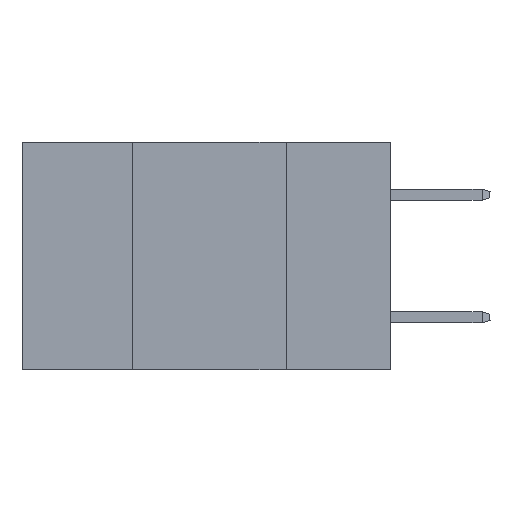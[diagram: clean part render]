
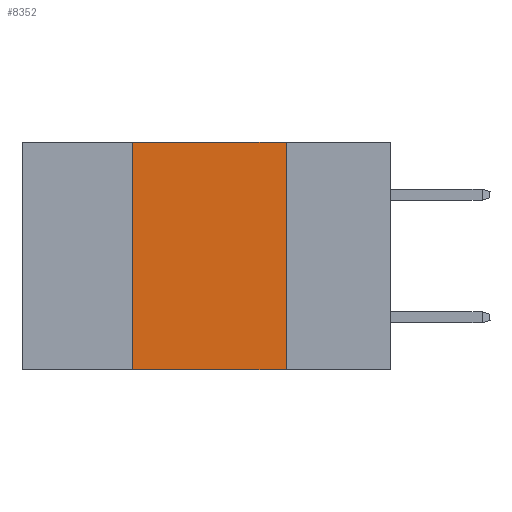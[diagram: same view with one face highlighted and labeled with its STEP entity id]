
A CAD part, left-side view. The second image highlights one B-rep face of the part: STEP entity #8352.
In plain terms, the highlighted planar face has unit normal (-1, 0, 0).
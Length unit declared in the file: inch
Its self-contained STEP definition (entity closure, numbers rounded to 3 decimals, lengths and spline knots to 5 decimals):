
#194 = ORIENTED_EDGE ( 'NONE', *, *, #8612, .T. ) ;
#572 = CARTESIAN_POINT ( 'NONE',  ( 0., 0.6, 0. ) ) ;
#630 = VECTOR ( 'NONE', #4818, 39.37008 ) ;
#926 = LINE ( 'NONE', #2051, #630 ) ;
#952 = VECTOR ( 'NONE', #7758, 39.37008 ) ;
#1507 = DIRECTION ( 'NONE',  ( 0., -1., 0. ) ) ;
#1665 = CARTESIAN_POINT ( 'NONE',  ( 0., 0.42, 0. ) ) ;
#1804 = AXIS2_PLACEMENT_3D ( 'NONE', #10772, #2562, #8501 ) ;
#1829 = CARTESIAN_POINT ( 'NONE',  ( 0., 0.17, 0. ) ) ;
#1857 = CARTESIAN_POINT ( 'NONE',  ( 0., 0.17, 0. ) ) ;
#2051 = CARTESIAN_POINT ( 'NONE',  ( 0., 0.6, -0.37 ) ) ;
#2395 = VECTOR ( 'NONE', #7905, 39.37008 ) ;
#2544 = VERTEX_POINT ( 'NONE', #1857 ) ;
#2562 = DIRECTION ( 'NONE',  ( 1., 0., 0. ) ) ;
#2824 = CARTESIAN_POINT ( 'NONE',  ( 0., 0.42, -0.37 ) ) ;
#2958 = CARTESIAN_POINT ( 'NONE',  ( 0., 0.17, -0.37 ) ) ;
#3360 = EDGE_LOOP ( 'NONE', ( #6223, #10893, #4802, #194 ) ) ;
#3455 = LINE ( 'NONE', #1665, #952 ) ;
#3553 = VECTOR ( 'NONE', #1507, 39.37008 ) ;
#4107 = FACE_OUTER_BOUND ( 'NONE', #3360, .T. ) ;
#4354 = VERTEX_POINT ( 'NONE', #2958 ) ;
#4670 = VERTEX_POINT ( 'NONE', #2824 ) ;
#4802 = ORIENTED_EDGE ( 'NONE', *, *, #7892, .F. ) ;
#4818 = DIRECTION ( 'NONE',  ( 0., -1., 0. ) ) ;
#5224 = CARTESIAN_POINT ( 'NONE',  ( 0., 0.42, 0. ) ) ;
#6177 = VERTEX_POINT ( 'NONE', #5224 ) ;
#6223 = ORIENTED_EDGE ( 'NONE', *, *, #7581, .F. ) ;
#6759 = LINE ( 'NONE', #1829, #2395 ) ;
#7581 = EDGE_CURVE ( 'NONE', #2544, #4354, #6759, .T. ) ;
#7758 = DIRECTION ( 'NONE',  ( 0., 0., 1. ) ) ;
#7892 = EDGE_CURVE ( 'NONE', #4670, #6177, #3455, .T. ) ;
#7905 = DIRECTION ( 'NONE',  ( 0., 0., -1. ) ) ;
#8352 = ADVANCED_FACE ( 'NONE', ( #4107 ), #8471, .F. ) ;
#8471 = PLANE ( 'NONE',  #1804 ) ;
#8501 = DIRECTION ( 'NONE',  ( 0., 0., -1. ) ) ;
#8612 = EDGE_CURVE ( 'NONE', #4670, #4354, #926, .T. ) ;
#9185 = EDGE_CURVE ( 'NONE', #6177, #2544, #10083, .T. ) ;
#10083 = LINE ( 'NONE', #572, #3553 ) ;
#10772 = CARTESIAN_POINT ( 'NONE',  ( 0., 0.6, 0. ) ) ;
#10893 = ORIENTED_EDGE ( 'NONE', *, *, #9185, .F. ) ;
